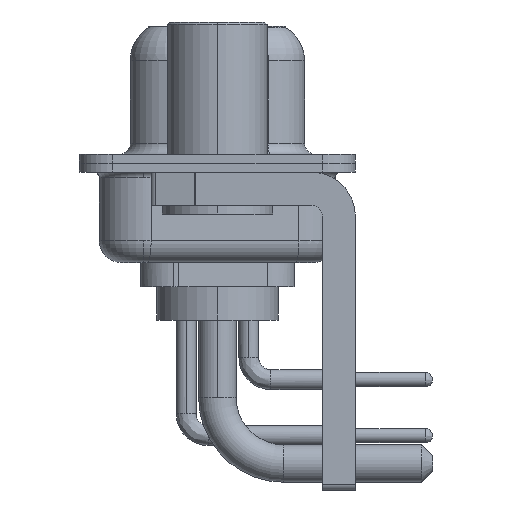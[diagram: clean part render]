
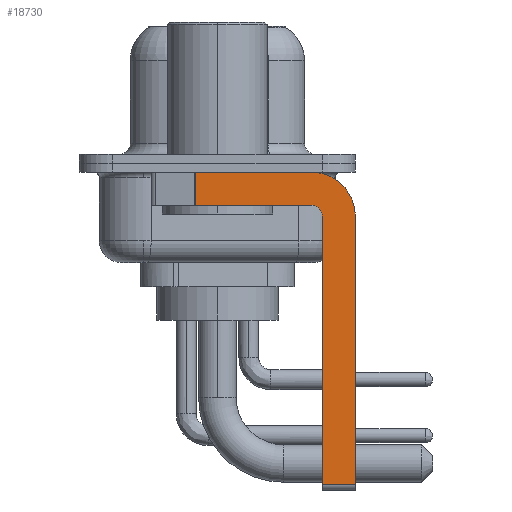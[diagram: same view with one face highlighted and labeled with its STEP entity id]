
A CAD part, left-side view. The second image highlights one B-rep face of the part: STEP entity #18730.
In plain terms, the highlighted planar face has unit normal (-1, 0, 0).
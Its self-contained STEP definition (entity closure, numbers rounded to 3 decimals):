
#164 = AXIS2_PLACEMENT_3D ( 'NONE', #10328, #20482, #22894 ) ;
#198 = CARTESIAN_POINT ( 'NONE',  ( -2.9, -6.25, -2.4 ) ) ;
#268 = EDGE_CURVE ( 'NONE', #13894, #11775, #9775, .T. ) ;
#396 = VECTOR ( 'NONE', #6246, 1000. ) ;
#536 = LINE ( 'NONE', #20661, #396 ) ;
#1636 = CARTESIAN_POINT ( 'NONE',  ( -2.9, -4.25, -1.9 ) ) ;
#1638 = DIRECTION ( 'NONE',  ( 0., 0., -1. ) ) ;
#1860 = DIRECTION ( 'NONE',  ( 1., 0., 0. ) ) ;
#2111 = CARTESIAN_POINT ( 'NONE',  ( -2.9, -4.25, -2.4 ) ) ;
#2937 = EDGE_CURVE ( 'NONE', #15727, #24416, #11637, .T. ) ;
#3014 = DIRECTION ( 'NONE',  ( 0., -1., 0. ) ) ;
#3065 = VECTOR ( 'NONE', #3014, 1000. ) ;
#3811 = ORIENTED_EDGE ( 'NONE', *, *, #2937, .F. ) ;
#4158 = CIRCLE ( 'NONE', #6275, 2. ) ;
#4246 = EDGE_CURVE ( 'NONE', #17844, #16590, #18546, .T. ) ;
#4578 = EDGE_CURVE ( 'NONE', #24416, #11775, #536, .T. ) ;
#5278 = EDGE_CURVE ( 'NONE', #13894, #23702, #18880, .T. ) ;
#6044 = CARTESIAN_POINT ( 'NONE',  ( -2.9, -4.25, -2.4 ) ) ;
#6246 = DIRECTION ( 'NONE',  ( 0., 1., 0. ) ) ;
#6275 = AXIS2_PLACEMENT_3D ( 'NONE', #6044, #24590, #14428 ) ;
#6502 = ORIENTED_EDGE ( 'NONE', *, *, #20958, .T. ) ;
#7650 = CARTESIAN_POINT ( 'NONE',  ( -2.9, 0.978, -1.9 ) ) ;
#8273 = PLANE ( 'NONE',  #18250 ) ;
#9502 = ORIENTED_EDGE ( 'NONE', *, *, #17906, .F. ) ;
#9758 = CARTESIAN_POINT ( 'NONE',  ( -2.9, -4.75, -14.8 ) ) ;
#9775 = LINE ( 'NONE', #7650, #15542 ) ;
#9990 = FACE_OUTER_BOUND ( 'NONE', #20732, .T. ) ;
#10328 = CARTESIAN_POINT ( 'NONE',  ( -2.9, -4.25, -2.4 ) ) ;
#10892 = CARTESIAN_POINT ( 'NONE',  ( -2.9, -4.75, -2.4 ) ) ;
#11601 = LINE ( 'NONE', #19749, #22985 ) ;
#11637 = CIRCLE ( 'NONE', #164, 0.5 ) ;
#11775 = VERTEX_POINT ( 'NONE', #24741 ) ;
#12323 = ORIENTED_EDGE ( 'NONE', *, *, #4246, .F. ) ;
#13003 = VECTOR ( 'NONE', #22566, 1000. ) ;
#13059 = ORIENTED_EDGE ( 'NONE', *, *, #18131, .F. ) ;
#13894 = VERTEX_POINT ( 'NONE', #25723 ) ;
#13969 = VECTOR ( 'NONE', #17263, 1000. ) ;
#14428 = DIRECTION ( 'NONE',  ( 0., 0., -1. ) ) ;
#15542 = VECTOR ( 'NONE', #1638, 1000. ) ;
#15727 = VERTEX_POINT ( 'NONE', #10892 ) ;
#16590 = VERTEX_POINT ( 'NONE', #22456 ) ;
#17263 = DIRECTION ( 'NONE',  ( 0., 0., 1. ) ) ;
#17265 = ORIENTED_EDGE ( 'NONE', *, *, #268, .T. ) ;
#17844 = VERTEX_POINT ( 'NONE', #198 ) ;
#17906 = EDGE_CURVE ( 'NONE', #23702, #17844, #4158, .T. ) ;
#18131 = EDGE_CURVE ( 'NONE', #21862, #15727, #19141, .T. ) ;
#18250 = AXIS2_PLACEMENT_3D ( 'NONE', #2111, #1860, #24279 ) ;
#18546 = LINE ( 'NONE', #20689, #13003 ) ;
#18730 = ADVANCED_FACE ( 'NONE', ( #9990 ), #8273, .F. ) ;
#18735 = ORIENTED_EDGE ( 'NONE', *, *, #5278, .F. ) ;
#18880 = LINE ( 'NONE', #25166, #3065 ) ;
#19141 = LINE ( 'NONE', #9758, #13969 ) ;
#19749 = CARTESIAN_POINT ( 'NONE',  ( -2.9, -4.25, -14.55 ) ) ;
#20269 = CARTESIAN_POINT ( 'NONE',  ( -2.9, -4.75, -14.55 ) ) ;
#20482 = DIRECTION ( 'NONE',  ( -1., 0., 0. ) ) ;
#20661 = CARTESIAN_POINT ( 'NONE',  ( -2.9, -4.25, -1.9 ) ) ;
#20689 = CARTESIAN_POINT ( 'NONE',  ( -2.9, -6.25, -2.4 ) ) ;
#20732 = EDGE_LOOP ( 'NONE', ( #18735, #17265, #25265, #3811, #13059, #6502, #12323, #9502 ) ) ;
#20958 = EDGE_CURVE ( 'NONE', #21862, #16590, #11601, .T. ) ;
#21862 = VERTEX_POINT ( 'NONE', #20269 ) ;
#22456 = CARTESIAN_POINT ( 'NONE',  ( -2.9, -6.25, -14.55 ) ) ;
#22566 = DIRECTION ( 'NONE',  ( 0., 0., -1. ) ) ;
#22894 = DIRECTION ( 'NONE',  ( 0., 0., 1. ) ) ;
#22985 = VECTOR ( 'NONE', #26001, 1000. ) ;
#23702 = VERTEX_POINT ( 'NONE', #24290 ) ;
#24279 = DIRECTION ( 'NONE',  ( 0., 0., -1. ) ) ;
#24290 = CARTESIAN_POINT ( 'NONE',  ( -2.9, -4.25, -0.4 ) ) ;
#24416 = VERTEX_POINT ( 'NONE', #1636 ) ;
#24590 = DIRECTION ( 'NONE',  ( 1., 0., 0. ) ) ;
#24741 = CARTESIAN_POINT ( 'NONE',  ( -2.9, 0.978, -1.9 ) ) ;
#25166 = CARTESIAN_POINT ( 'NONE',  ( -2.9, 3., -0.4 ) ) ;
#25265 = ORIENTED_EDGE ( 'NONE', *, *, #4578, .F. ) ;
#25723 = CARTESIAN_POINT ( 'NONE',  ( -2.9, 0.978, -0.4 ) ) ;
#26001 = DIRECTION ( 'NONE',  ( 0., -1., 0. ) ) ;
